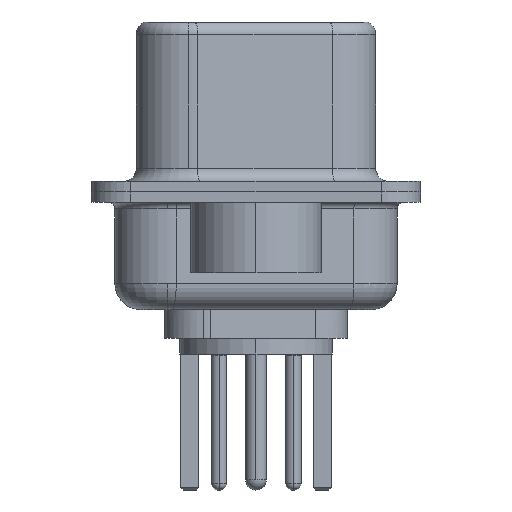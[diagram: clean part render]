
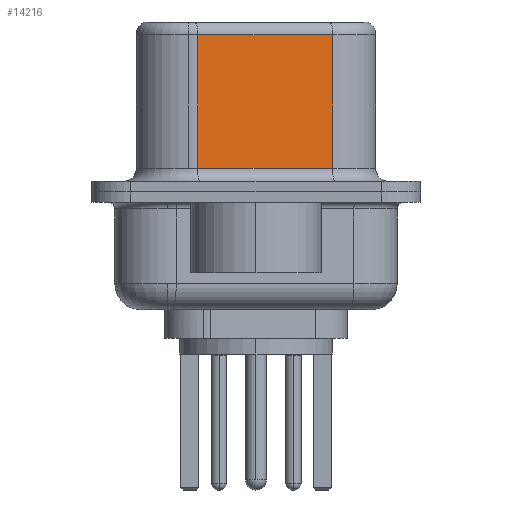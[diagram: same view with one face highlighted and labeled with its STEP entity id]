
A CAD part, left-side view. The second image highlights one B-rep face of the part: STEP entity #14216.
In plain terms, the highlighted planar face has unit normal (-0.985, -0.174, 0).
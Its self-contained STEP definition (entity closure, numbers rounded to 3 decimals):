
#740 = DIRECTION ( 'NONE',  ( 0.985, 0.174, 0. ) ) ;
#2170 = CARTESIAN_POINT ( 'NONE',  ( 4.585, -2.927, 0.9 ) ) ;
#2178 = ORIENTED_EDGE ( 'NONE', *, *, #19321, .T. ) ;
#2423 = ORIENTED_EDGE ( 'NONE', *, *, #4050, .T. ) ;
#2668 = EDGE_CURVE ( 'NONE', #3974, #15240, #15394, .T. ) ;
#2670 = CARTESIAN_POINT ( 'NONE',  ( 3.675, 2.233, 6.52 ) ) ;
#2732 = AXIS2_PLACEMENT_3D ( 'NONE', #9881, #740, #11413 ) ;
#2862 = ORIENTED_EDGE ( 'NONE', *, *, #12535, .F. ) ;
#3055 = VECTOR ( 'NONE', #16714, 1000. ) ;
#3440 = VERTEX_POINT ( 'NONE', #19207 ) ;
#3974 = VERTEX_POINT ( 'NONE', #18841 ) ;
#4050 = EDGE_CURVE ( 'NONE', #15240, #3440, #7588, .T. ) ;
#6543 = CARTESIAN_POINT ( 'NONE',  ( 4.585, -2.927, 6.02 ) ) ;
#6732 = FACE_OUTER_BOUND ( 'NONE', #18846, .T. ) ;
#7588 = LINE ( 'NONE', #2670, #8101 ) ;
#8101 = VECTOR ( 'NONE', #11963, 1000. ) ;
#8360 = PLANE ( 'NONE',  #2732 ) ;
#8905 = VECTOR ( 'NONE', #10481, 1000. ) ;
#9881 = CARTESIAN_POINT ( 'NONE',  ( 4.585, -2.927, 6.52 ) ) ;
#10413 = CARTESIAN_POINT ( 'NONE',  ( 4.585, -2.927, 6.52 ) ) ;
#10481 = DIRECTION ( 'NONE',  ( 0., 0., -1. ) ) ;
#11413 = DIRECTION ( 'NONE',  ( -0.174, 0.985, 0. ) ) ;
#11584 = LINE ( 'NONE', #2170, #19190 ) ;
#11963 = DIRECTION ( 'NONE',  ( 0., 0., -1. ) ) ;
#12348 = CARTESIAN_POINT ( 'NONE',  ( 3.675, 2.233, 6.02 ) ) ;
#12535 = EDGE_CURVE ( 'NONE', #3974, #14681, #16972, .T. ) ;
#14216 = ADVANCED_FACE ( 'NONE', ( #6732 ), #8360, .F. ) ;
#14681 = VERTEX_POINT ( 'NONE', #15707 ) ;
#15240 = VERTEX_POINT ( 'NONE', #12348 ) ;
#15394 = LINE ( 'NONE', #6543, #3055 ) ;
#15707 = CARTESIAN_POINT ( 'NONE',  ( 4.585, -2.927, 0.9 ) ) ;
#15739 = ORIENTED_EDGE ( 'NONE', *, *, #2668, .T. ) ;
#16714 = DIRECTION ( 'NONE',  ( -0.174, 0.985, 0. ) ) ;
#16972 = LINE ( 'NONE', #10413, #8905 ) ;
#17341 = DIRECTION ( 'NONE',  ( 0.174, -0.985, 0. ) ) ;
#18841 = CARTESIAN_POINT ( 'NONE',  ( 4.585, -2.927, 6.02 ) ) ;
#18846 = EDGE_LOOP ( 'NONE', ( #2862, #15739, #2423, #2178 ) ) ;
#19190 = VECTOR ( 'NONE', #17341, 1000. ) ;
#19207 = CARTESIAN_POINT ( 'NONE',  ( 3.675, 2.233, 0.9 ) ) ;
#19321 = EDGE_CURVE ( 'NONE', #3440, #14681, #11584, .T. ) ;
